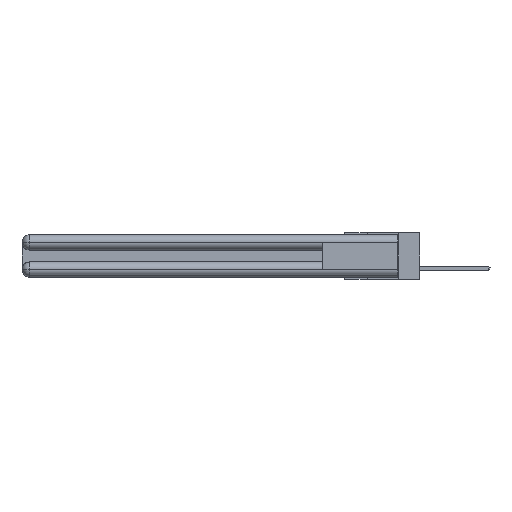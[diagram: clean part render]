
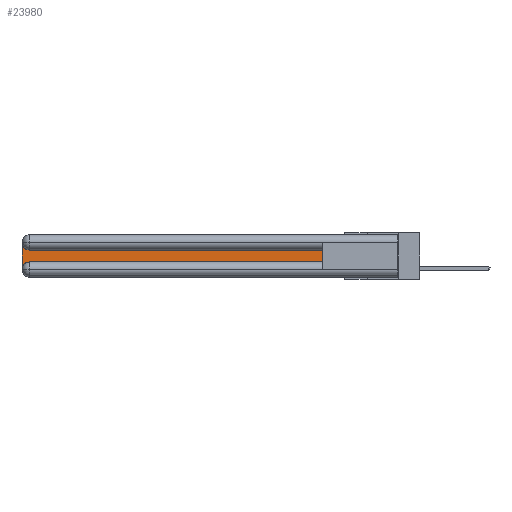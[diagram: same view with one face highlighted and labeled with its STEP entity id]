
A CAD part, left-side view. The second image highlights one B-rep face of the part: STEP entity #23980.
In plain terms, the highlighted planar face has unit normal (-1, 0, 0).
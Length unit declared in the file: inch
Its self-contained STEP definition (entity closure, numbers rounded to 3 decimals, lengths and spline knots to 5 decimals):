
#180 = EDGE_CURVE ( 'NONE', #25198, #28516, #20611, .T. ) ;
#740 = FACE_OUTER_BOUND ( 'NONE', #16296, .T. ) ;
#1183 = DIRECTION ( 'NONE',  ( 0., 0., -1. ) ) ;
#1811 = DIRECTION ( 'NONE',  ( 0., -1., 0. ) ) ;
#2328 = EDGE_CURVE ( 'NONE', #30937, #25198, #26045, .T. ) ;
#2408 = VECTOR ( 'NONE', #1811, 39.37008 ) ;
#2858 = ORIENTED_EDGE ( 'NONE', *, *, #19382, .T. ) ;
#3339 = EDGE_CURVE ( 'NONE', #11523, #15960, #8785, .T. ) ;
#3761 = VECTOR ( 'NONE', #1183, 39.37008 ) ;
#4508 = AXIS2_PLACEMENT_3D ( 'NONE', #26902, #17319, #21937 ) ;
#4733 = EDGE_CURVE ( 'NONE', #13667, #30937, #27701, .T. ) ;
#5170 = CIRCLE ( 'NONE', #4508, 0.06 ) ;
#7108 = CARTESIAN_POINT ( 'NONE',  ( 0.075, 3., -0.0625 ) ) ;
#7375 = CARTESIAN_POINT ( 'NONE',  ( 0.075, 2.94, -0.2175 ) ) ;
#7917 = CARTESIAN_POINT ( 'NONE',  ( 0.075, 3., -0.1225 ) ) ;
#8785 = LINE ( 'NONE', #25828, #2408 ) ;
#10595 = CARTESIAN_POINT ( 'NONE',  ( 0.075, 0.6, -0.2175 ) ) ;
#11523 = VERTEX_POINT ( 'NONE', #7375 ) ;
#13206 = DIRECTION ( 'NONE',  ( 0., 0., 1. ) ) ;
#13667 = VERTEX_POINT ( 'NONE', #28445 ) ;
#15222 = VECTOR ( 'NONE', #13206, 39.37008 ) ;
#15244 = PLANE ( 'NONE',  #17024 ) ;
#15960 = VERTEX_POINT ( 'NONE', #21438 ) ;
#16296 = EDGE_LOOP ( 'NONE', ( #25633, #25368, #24115, #23116, #23272, #2858 ) ) ;
#17024 = AXIS2_PLACEMENT_3D ( 'NONE', #7917, #29402, #24867 ) ;
#17319 = DIRECTION ( 'NONE',  ( 1., 0., 0. ) ) ;
#18431 = VECTOR ( 'NONE', #27688, 39.37008 ) ;
#18876 = CARTESIAN_POINT ( 'NONE',  ( 0.075, 2.94, -0.0625 ) ) ;
#19382 = EDGE_CURVE ( 'NONE', #15960, #13667, #24173, .T. ) ;
#20241 = CARTESIAN_POINT ( 'NONE',  ( 0.075, 3., -0.2175 ) ) ;
#20611 = LINE ( 'NONE', #20241, #3761 ) ;
#21438 = CARTESIAN_POINT ( 'NONE',  ( 0.075, 0.6, -0.2175 ) ) ;
#21937 = DIRECTION ( 'NONE',  ( 0., 0., -1. ) ) ;
#23054 = CARTESIAN_POINT ( 'NONE',  ( 0.075, 0.6, -0.1225 ) ) ;
#23116 = ORIENTED_EDGE ( 'NONE', *, *, #30556, .T. ) ;
#23272 = ORIENTED_EDGE ( 'NONE', *, *, #3339, .T. ) ;
#23478 = AXIS2_PLACEMENT_3D ( 'NONE', #18876, #23641, #28077 ) ;
#23641 = DIRECTION ( 'NONE',  ( 1., 0., 0. ) ) ;
#23980 = ADVANCED_FACE ( 'NONE', ( #740 ), #15244, .F. ) ;
#24115 = ORIENTED_EDGE ( 'NONE', *, *, #180, .T. ) ;
#24173 = LINE ( 'NONE', #10595, #15222 ) ;
#24867 = DIRECTION ( 'NONE',  ( 0., 0., -1. ) ) ;
#25198 = VERTEX_POINT ( 'NONE', #7108 ) ;
#25368 = ORIENTED_EDGE ( 'NONE', *, *, #2328, .T. ) ;
#25633 = ORIENTED_EDGE ( 'NONE', *, *, #4733, .T. ) ;
#25828 = CARTESIAN_POINT ( 'NONE',  ( 0.075, 0.6, -0.2175 ) ) ;
#26045 = CIRCLE ( 'NONE', #23478, 0.06 ) ;
#26902 = CARTESIAN_POINT ( 'NONE',  ( 0.075, 2.94, -0.2775 ) ) ;
#27688 = DIRECTION ( 'NONE',  ( 0., 1., 0. ) ) ;
#27701 = LINE ( 'NONE', #23054, #18431 ) ;
#28077 = DIRECTION ( 'NONE',  ( 0., 0., -1. ) ) ;
#28317 = CARTESIAN_POINT ( 'NONE',  ( 0.075, 3., -0.2775 ) ) ;
#28445 = CARTESIAN_POINT ( 'NONE',  ( 0.075, 0.6, -0.1225 ) ) ;
#28516 = VERTEX_POINT ( 'NONE', #28317 ) ;
#29402 = DIRECTION ( 'NONE',  ( 1., 0., 0. ) ) ;
#30102 = CARTESIAN_POINT ( 'NONE',  ( 0.075, 2.94, -0.1225 ) ) ;
#30556 = EDGE_CURVE ( 'NONE', #28516, #11523, #5170, .T. ) ;
#30937 = VERTEX_POINT ( 'NONE', #30102 ) ;
